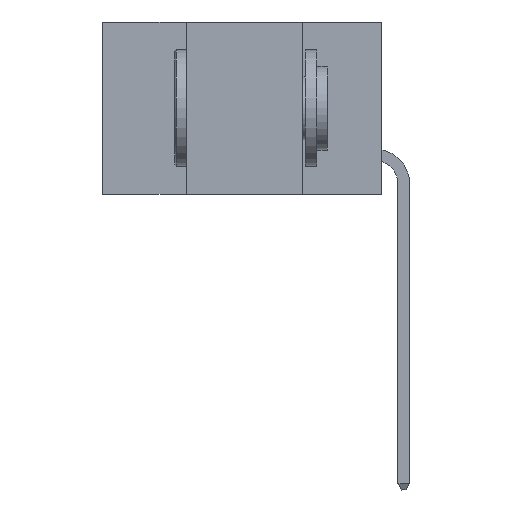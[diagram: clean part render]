
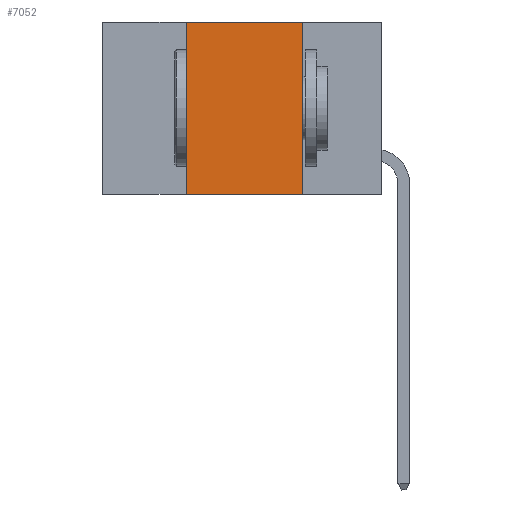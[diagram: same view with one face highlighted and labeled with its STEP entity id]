
A CAD part, left-side view. The second image highlights one B-rep face of the part: STEP entity #7052.
In plain terms, the highlighted planar face has unit normal (-1, 0, 0).
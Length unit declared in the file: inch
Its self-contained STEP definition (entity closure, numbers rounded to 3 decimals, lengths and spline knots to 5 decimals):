
#697 = DIRECTION ( 'NONE',  ( 0., 0., -1. ) ) ;
#713 = DIRECTION ( 'NONE',  ( 1., 0., 0. ) ) ;
#734 = PLANE ( 'NONE',  #991 ) ;
#838 = VERTEX_POINT ( 'NONE', #1100 ) ;
#991 = AXIS2_PLACEMENT_3D ( 'NONE', #1080, #713, #697 ) ;
#1080 = CARTESIAN_POINT ( 'NONE',  ( 0., 0.6, 0. ) ) ;
#1100 = CARTESIAN_POINT ( 'NONE',  ( 0., 0.17, 0. ) ) ;
#1240 = CARTESIAN_POINT ( 'NONE',  ( 0., 0.42, 0. ) ) ;
#1868 = CARTESIAN_POINT ( 'NONE',  ( 0., 0.17, -0.37 ) ) ;
#2302 = CARTESIAN_POINT ( 'NONE',  ( 0., 0.6, -0.37 ) ) ;
#2306 = LINE ( 'NONE', #9175, #10500 ) ;
#2659 = VECTOR ( 'NONE', #10490, 39.37008 ) ;
#2726 = CARTESIAN_POINT ( 'NONE',  ( 0., 0.17, 0. ) ) ;
#2913 = VECTOR ( 'NONE', #2931, 39.37008 ) ;
#2931 = DIRECTION ( 'NONE',  ( 0., -1., 0. ) ) ;
#3193 = VERTEX_POINT ( 'NONE', #6604 ) ;
#3335 = FACE_OUTER_BOUND ( 'NONE', #5494, .T. ) ;
#3469 = EDGE_CURVE ( 'NONE', #4212, #838, #2306, .T. ) ;
#3475 = LINE ( 'NONE', #7714, #11422 ) ;
#3476 = LINE ( 'NONE', #2302, #2913 ) ;
#3955 = ORIENTED_EDGE ( 'NONE', *, *, #3469, .F. ) ;
#4212 = VERTEX_POINT ( 'NONE', #1240 ) ;
#4794 = LINE ( 'NONE', #2726, #2659 ) ;
#4857 = EDGE_CURVE ( 'NONE', #3193, #4212, #3475, .T. ) ;
#5494 = EDGE_LOOP ( 'NONE', ( #9902, #3955, #10294, #11126 ) ) ;
#6140 = DIRECTION ( 'NONE',  ( 0., 0., 1. ) ) ;
#6604 = CARTESIAN_POINT ( 'NONE',  ( 0., 0.42, -0.37 ) ) ;
#6935 = EDGE_CURVE ( 'NONE', #3193, #10733, #3476, .T. ) ;
#7052 = ADVANCED_FACE ( 'NONE', ( #3335 ), #734, .F. ) ;
#7714 = CARTESIAN_POINT ( 'NONE',  ( 0., 0.42, 0. ) ) ;
#9175 = CARTESIAN_POINT ( 'NONE',  ( 0., 0.6, 0. ) ) ;
#9803 = DIRECTION ( 'NONE',  ( 0., -1., 0. ) ) ;
#9902 = ORIENTED_EDGE ( 'NONE', *, *, #10607, .F. ) ;
#10294 = ORIENTED_EDGE ( 'NONE', *, *, #4857, .F. ) ;
#10490 = DIRECTION ( 'NONE',  ( 0., 0., -1. ) ) ;
#10500 = VECTOR ( 'NONE', #9803, 39.37008 ) ;
#10607 = EDGE_CURVE ( 'NONE', #838, #10733, #4794, .T. ) ;
#10733 = VERTEX_POINT ( 'NONE', #1868 ) ;
#11126 = ORIENTED_EDGE ( 'NONE', *, *, #6935, .T. ) ;
#11422 = VECTOR ( 'NONE', #6140, 39.37008 ) ;
